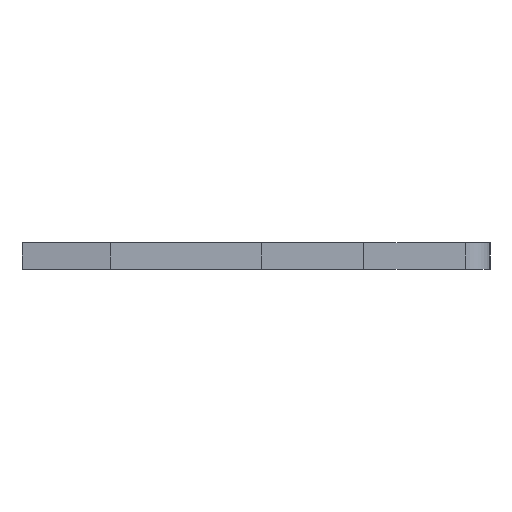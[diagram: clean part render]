
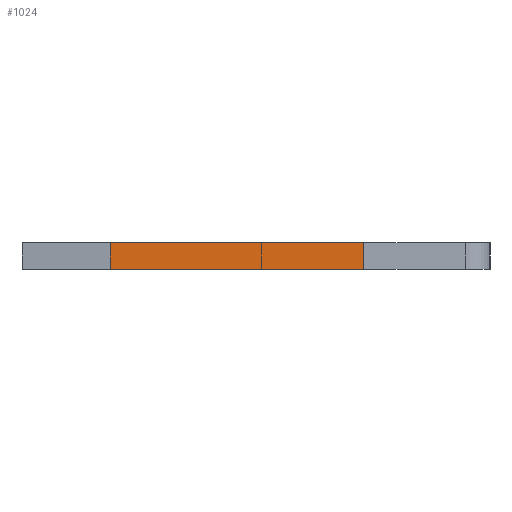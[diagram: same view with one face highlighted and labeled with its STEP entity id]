
A CAD part, left-side view. The second image highlights one B-rep face of the part: STEP entity #1024.
In plain terms, the highlighted face is planar.
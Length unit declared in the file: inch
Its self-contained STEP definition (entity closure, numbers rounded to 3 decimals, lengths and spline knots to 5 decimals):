
#44 = CARTESIAN_POINT ( 'NONE',  ( -0.013, 0.146, -0.0575 ) ) ;
#69 = ORIENTED_EDGE ( 'NONE', *, *, #2323, .T. ) ;
#259 = DIRECTION ( 'NONE',  ( 0., 1., 0. ) ) ;
#302 = DIRECTION ( 'NONE',  ( 0., 0., 1. ) ) ;
#354 = VERTEX_POINT ( 'NONE', #1150 ) ;
#381 = VERTEX_POINT ( 'NONE', #1921 ) ;
#421 = EDGE_LOOP ( 'NONE', ( #69, #1752, #1965, #1123 ) ) ;
#468 = VECTOR ( 'NONE', #1721, 39.37008 ) ;
#644 = EDGE_CURVE ( 'NONE', #354, #2352, #2047, .T. ) ;
#748 = CARTESIAN_POINT ( 'NONE',  ( 0.013, 0.146, -0.0575 ) ) ;
#850 = PLANE ( 'NONE',  #1398 ) ;
#875 = VECTOR ( 'NONE', #2271, 39.37008 ) ;
#912 = LINE ( 'NONE', #44, #1042 ) ;
#968 = LINE ( 'NONE', #1928, #468 ) ;
#1024 = ADVANCED_FACE ( 'NONE', ( #1811 ), #850, .F. ) ;
#1042 = VECTOR ( 'NONE', #1563, 39.37008 ) ;
#1098 = CARTESIAN_POINT ( 'NONE',  ( -0.013, -0.099, -0.0575 ) ) ;
#1123 = ORIENTED_EDGE ( 'NONE', *, *, #2306, .T. ) ;
#1139 = VECTOR ( 'NONE', #259, 39.37008 ) ;
#1150 = CARTESIAN_POINT ( 'NONE',  ( 0.013, -0.099, -0.0575 ) ) ;
#1231 = VERTEX_POINT ( 'NONE', #1098 ) ;
#1248 = CARTESIAN_POINT ( 'NONE',  ( 0.013, 0.146, -0.0575 ) ) ;
#1394 = LINE ( 'NONE', #748, #875 ) ;
#1398 = AXIS2_PLACEMENT_3D ( 'NONE', #1248, #302, #2199 ) ;
#1452 = EDGE_CURVE ( 'NONE', #2352, #381, #1394, .T. ) ;
#1563 = DIRECTION ( 'NONE',  ( 0., 1., 0. ) ) ;
#1721 = DIRECTION ( 'NONE',  ( -1., 0., 0. ) ) ;
#1752 = ORIENTED_EDGE ( 'NONE', *, *, #1452, .F. ) ;
#1811 = FACE_OUTER_BOUND ( 'NONE', #421, .T. ) ;
#1908 = CARTESIAN_POINT ( 'NONE',  ( 0.013, 0.146, -0.0575 ) ) ;
#1921 = CARTESIAN_POINT ( 'NONE',  ( -0.013, 0.146, -0.0575 ) ) ;
#1928 = CARTESIAN_POINT ( 'NONE',  ( 0.013, -0.099, -0.0575 ) ) ;
#1938 = CARTESIAN_POINT ( 'NONE',  ( 0.013, 0.146, -0.0575 ) ) ;
#1965 = ORIENTED_EDGE ( 'NONE', *, *, #644, .F. ) ;
#2047 = LINE ( 'NONE', #1938, #1139 ) ;
#2199 = DIRECTION ( 'NONE',  ( 1., 0., 0. ) ) ;
#2271 = DIRECTION ( 'NONE',  ( -1., 0., 0. ) ) ;
#2306 = EDGE_CURVE ( 'NONE', #354, #1231, #968, .T. ) ;
#2323 = EDGE_CURVE ( 'NONE', #1231, #381, #912, .T. ) ;
#2352 = VERTEX_POINT ( 'NONE', #1908 ) ;
